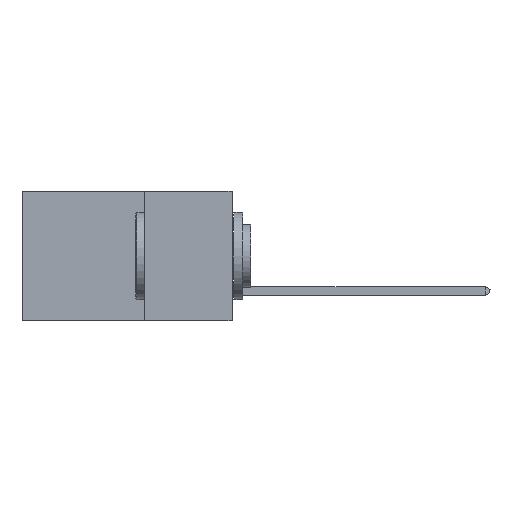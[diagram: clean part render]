
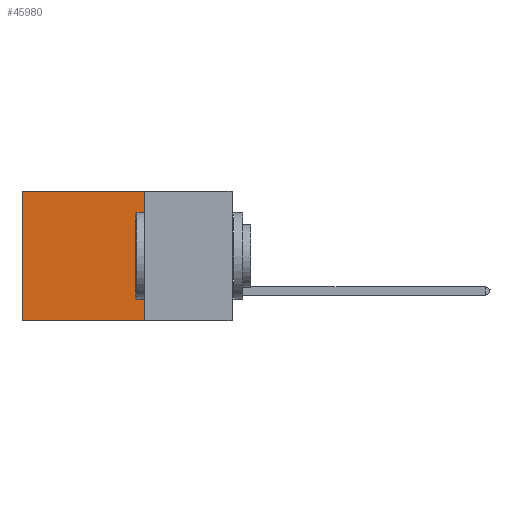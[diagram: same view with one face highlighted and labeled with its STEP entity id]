
A CAD part, left-side view. The second image highlights one B-rep face of the part: STEP entity #45980.
In plain terms, the highlighted planar face has unit normal (-1, 0, 0).
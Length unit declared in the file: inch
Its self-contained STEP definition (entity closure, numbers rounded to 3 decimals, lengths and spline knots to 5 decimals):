
#730 = LINE ( 'NONE', #25216, #39056 ) ;
#5051 = CARTESIAN_POINT ( 'NONE',  ( 0.2875, 0.25, 0. ) ) ;
#7543 = CARTESIAN_POINT ( 'NONE',  ( 0.2875, 0.25, -0.37 ) ) ;
#10451 = LINE ( 'NONE', #21571, #41181 ) ;
#11161 = CARTESIAN_POINT ( 'NONE',  ( 0.2875, 0.6, 0. ) ) ;
#12377 = ORIENTED_EDGE ( 'NONE', *, *, #47079, .F. ) ;
#12995 = VERTEX_POINT ( 'NONE', #21532 ) ;
#13022 = DIRECTION ( 'NONE',  ( 1., 0., 0. ) ) ;
#16861 = DIRECTION ( 'NONE',  ( 0., 1., 0. ) ) ;
#18435 = CARTESIAN_POINT ( 'NONE',  ( 0.2875, 0.25, 0. ) ) ;
#20753 = EDGE_CURVE ( 'NONE', #33448, #12995, #730, .T. ) ;
#21079 = CARTESIAN_POINT ( 'NONE',  ( 0.2875, 0.25, 0. ) ) ;
#21532 = CARTESIAN_POINT ( 'NONE',  ( 0.2875, 0.6, -0.37 ) ) ;
#21571 = CARTESIAN_POINT ( 'NONE',  ( 0.2875, 0.6, 0. ) ) ;
#21653 = VECTOR ( 'NONE', #34578, 39.37008 ) ;
#22133 = EDGE_LOOP ( 'NONE', ( #40649, #28012, #12377, #34123 ) ) ;
#24774 = LINE ( 'NONE', #21079, #35783 ) ;
#25216 = CARTESIAN_POINT ( 'NONE',  ( 0.2875, 0.25, -0.37 ) ) ;
#26176 = DIRECTION ( 'NONE',  ( 0., 1., 0. ) ) ;
#28012 = ORIENTED_EDGE ( 'NONE', *, *, #20753, .F. ) ;
#29316 = DIRECTION ( 'NONE',  ( 0., 0., -1. ) ) ;
#30117 = VERTEX_POINT ( 'NONE', #11161 ) ;
#31316 = DIRECTION ( 'NONE',  ( 0., 0., -1. ) ) ;
#33448 = VERTEX_POINT ( 'NONE', #7543 ) ;
#34123 = ORIENTED_EDGE ( 'NONE', *, *, #34458, .T. ) ;
#34458 = EDGE_CURVE ( 'NONE', #42718, #30117, #24774, .T. ) ;
#34578 = DIRECTION ( 'NONE',  ( 0., 0., -1. ) ) ;
#34965 = LINE ( 'NONE', #45769, #21653 ) ;
#35783 = VECTOR ( 'NONE', #16861, 39.37008 ) ;
#37981 = FACE_OUTER_BOUND ( 'NONE', #22133, .T. ) ;
#38495 = EDGE_CURVE ( 'NONE', #30117, #12995, #10451, .T. ) ;
#38778 = PLANE ( 'NONE',  #42161 ) ;
#39056 = VECTOR ( 'NONE', #26176, 39.37008 ) ;
#40649 = ORIENTED_EDGE ( 'NONE', *, *, #38495, .T. ) ;
#41181 = VECTOR ( 'NONE', #29316, 39.37008 ) ;
#42161 = AXIS2_PLACEMENT_3D ( 'NONE', #5051, #13022, #31316 ) ;
#42718 = VERTEX_POINT ( 'NONE', #18435 ) ;
#45769 = CARTESIAN_POINT ( 'NONE',  ( 0.2875, 0.25, 0. ) ) ;
#45980 = ADVANCED_FACE ( 'NONE', ( #37981 ), #38778, .F. ) ;
#47079 = EDGE_CURVE ( 'NONE', #42718, #33448, #34965, .T. ) ;
